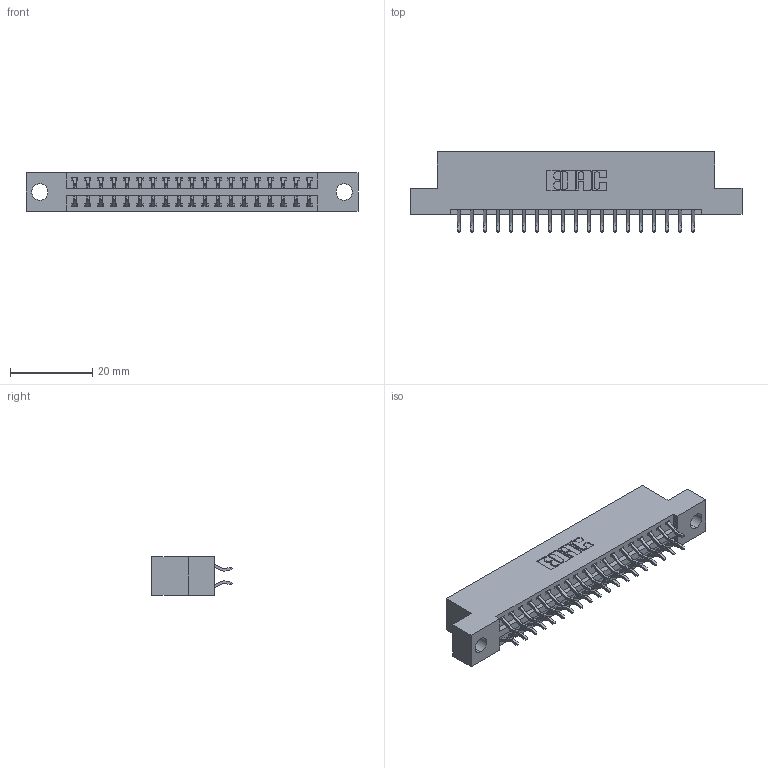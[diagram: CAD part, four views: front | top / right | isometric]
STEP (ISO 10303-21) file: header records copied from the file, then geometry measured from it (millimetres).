
FILE_DESCRIPTION (( 'STEP AP203' ), '1' );
FILE_NAME ('396-038-556-204.STEP', '2019-10-30T08:22:46', ( '' ), ( '' ), 'SwSTEP 2.0', 'SolidWorks 2016', '' );
FILE_SCHEMA (( 'CONFIG_CONTROL_DESIGN' ));
Length unit declared in the file: inch
Products named in the file (3): 396-038-556-204; 345-292-001_556 Tail; 346 Part_Flush Mounting Lugs - 0.156 Dia-TH
Assembly tree (39 placements, depth 2):
  396-038-556-204
    346 Part_Flush Mounting Lugs - 0.156 Dia-TH
    345-292-001_556 Tail  x38
Bounding box: 80.9 x 19.57 x 9.4 mm (x, y, z)
Volume: 7620.7 mm3; surface area: 9891.7 mm2
Topology: 39 solids, 39 shells, 2326 faces, 6903 edges, 4550 vertices
Faces by surface type: plane 1558, cylinder 768
Entity records: 15719 total; most frequent: CARTESIAN_POINT 2636, ORIENTED_EDGE 2558, DIRECTION 2363, EDGE_CURVE 1279, VECTOR 1063, LINE 1063, VERTEX_POINT 850, AXIS2_PLACEMENT_3D 650
